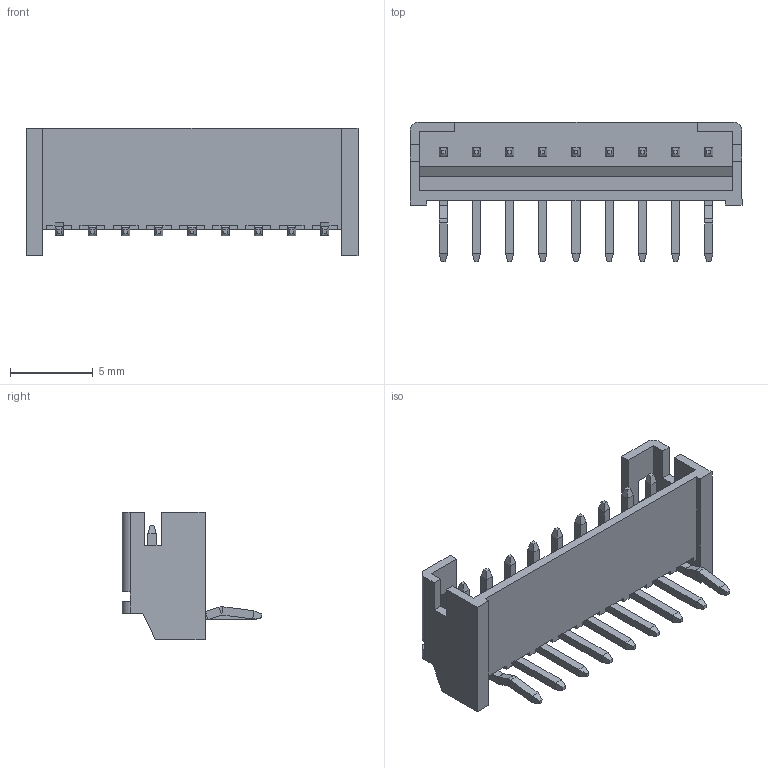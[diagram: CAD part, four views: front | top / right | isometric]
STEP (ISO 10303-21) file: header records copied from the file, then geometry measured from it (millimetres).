
FILE_DESCRIPTION (( 'STEP AP203' ), '1' );
FILE_NAME ('140-509-415-000.STEP', '2020-03-31T19:43:55', ( '' ), ( '' ), 'SwSTEP 2.0', 'SolidWorks 2016', '' );
FILE_SCHEMA (( 'CONFIG_CONTROL_DESIGN' ));
Length unit declared in the file: millimetre
Products named in the file (4): RA Housing_509; 140-509-415-000; RA Contact_Kink; RA Contact_Str
Assembly tree (10 placements, depth 2):
  140-509-415-000
    RA Housing_509
    RA Contact_Kink  x2
    RA Contact_Str  x7
Bounding box: 20 x 8.41 x 7.7 mm (x, y, z)
Volume: 239.1 mm3; surface area: 879 mm2
Topology: 10 solids, 10 shells, 349 faces, 813 edges, 482 vertices
Faces by surface type: plane 319, cylinder 30
Entity records: 6057 total; most frequent: CARTESIAN_POINT 963, ORIENTED_EDGE 946, DIRECTION 881, EDGE_CURVE 473, LINE 449, VECTOR 449, VERTEX_POINT 298, AXIS2_PLACEMENT_3D 216
